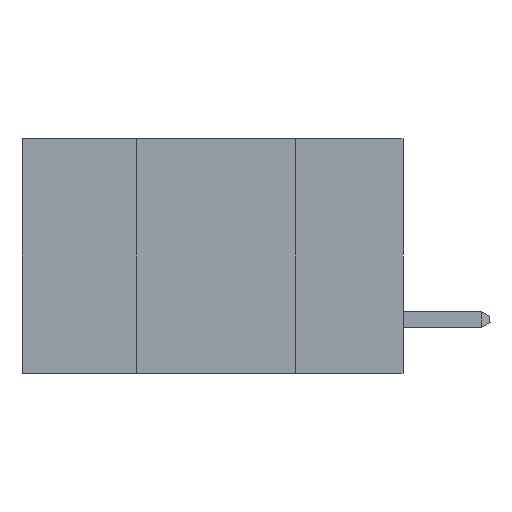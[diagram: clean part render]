
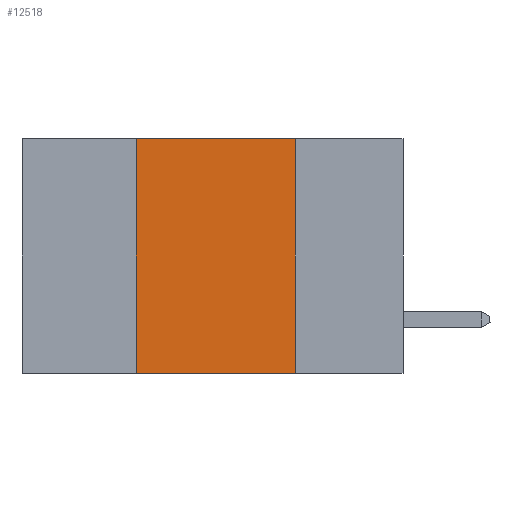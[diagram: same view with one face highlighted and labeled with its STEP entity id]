
A CAD part, left-side view. The second image highlights one B-rep face of the part: STEP entity #12518.
In plain terms, the highlighted planar face has unit normal (-1, 0, 0).
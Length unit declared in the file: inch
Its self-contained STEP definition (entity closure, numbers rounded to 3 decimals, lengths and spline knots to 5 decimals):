
#43 = VERTEX_POINT ( 'NONE', #1598 ) ;
#1598 = CARTESIAN_POINT ( 'NONE',  ( 0., 0.42, -0.37 ) ) ;
#1733 = EDGE_CURVE ( 'NONE', #43, #34362, #32532, .T. ) ;
#3321 = EDGE_LOOP ( 'NONE', ( #23963, #8838, #21999, #21744 ) ) ;
#4286 = VECTOR ( 'NONE', #9829, 39.37008 ) ;
#6029 = VECTOR ( 'NONE', #18048, 39.37008 ) ;
#7938 = AXIS2_PLACEMENT_3D ( 'NONE', #14823, #24441, #17368 ) ;
#8838 = ORIENTED_EDGE ( 'NONE', *, *, #15737, .F. ) ;
#9515 = CARTESIAN_POINT ( 'NONE',  ( 0., 0.6, -0.37 ) ) ;
#9829 = DIRECTION ( 'NONE',  ( 0., -1., 0. ) ) ;
#9838 = VECTOR ( 'NONE', #25266, 39.37008 ) ;
#10067 = CARTESIAN_POINT ( 'NONE',  ( 0., 0.6, 0. ) ) ;
#10158 = FACE_OUTER_BOUND ( 'NONE', #3321, .T. ) ;
#12518 = ADVANCED_FACE ( 'NONE', ( #10158 ), #16524, .F. ) ;
#12750 = DIRECTION ( 'NONE',  ( 0., -1., 0. ) ) ;
#13379 = LINE ( 'NONE', #15302, #6029 ) ;
#14823 = CARTESIAN_POINT ( 'NONE',  ( 0., 0.6, 0. ) ) ;
#15302 = CARTESIAN_POINT ( 'NONE',  ( 0., 0.17, 0. ) ) ;
#15737 = EDGE_CURVE ( 'NONE', #34362, #34514, #19267, .T. ) ;
#16524 = PLANE ( 'NONE',  #7938 ) ;
#17368 = DIRECTION ( 'NONE',  ( 0., 0., -1. ) ) ;
#18048 = DIRECTION ( 'NONE',  ( 0., 0., -1. ) ) ;
#19267 = LINE ( 'NONE', #10067, #4286 ) ;
#20846 = EDGE_CURVE ( 'NONE', #34514, #26506, #13379, .T. ) ;
#21744 = ORIENTED_EDGE ( 'NONE', *, *, #22730, .T. ) ;
#21999 = ORIENTED_EDGE ( 'NONE', *, *, #1733, .F. ) ;
#22277 = CARTESIAN_POINT ( 'NONE',  ( 0., 0.42, 0. ) ) ;
#22730 = EDGE_CURVE ( 'NONE', #43, #26506, #33617, .T. ) ;
#23963 = ORIENTED_EDGE ( 'NONE', *, *, #20846, .F. ) ;
#24441 = DIRECTION ( 'NONE',  ( 1., 0., 0. ) ) ;
#25266 = DIRECTION ( 'NONE',  ( 0., 0., 1. ) ) ;
#26469 = CARTESIAN_POINT ( 'NONE',  ( 0., 0.42, 0. ) ) ;
#26506 = VERTEX_POINT ( 'NONE', #32874 ) ;
#31486 = VECTOR ( 'NONE', #12750, 39.37008 ) ;
#32532 = LINE ( 'NONE', #22277, #9838 ) ;
#32874 = CARTESIAN_POINT ( 'NONE',  ( 0., 0.17, -0.37 ) ) ;
#33617 = LINE ( 'NONE', #9515, #31486 ) ;
#34362 = VERTEX_POINT ( 'NONE', #26469 ) ;
#34514 = VERTEX_POINT ( 'NONE', #34956 ) ;
#34956 = CARTESIAN_POINT ( 'NONE',  ( 0., 0.17, 0. ) ) ;
